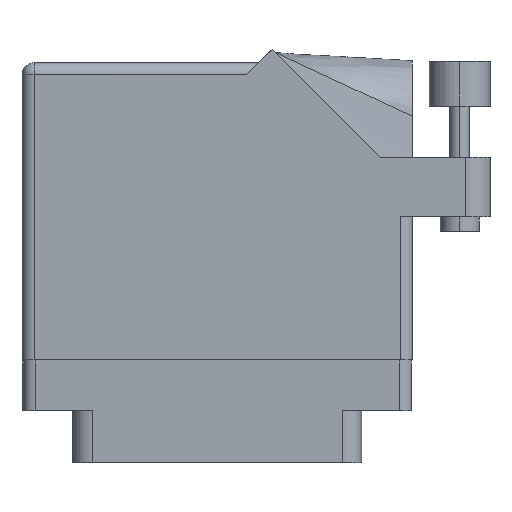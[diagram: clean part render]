
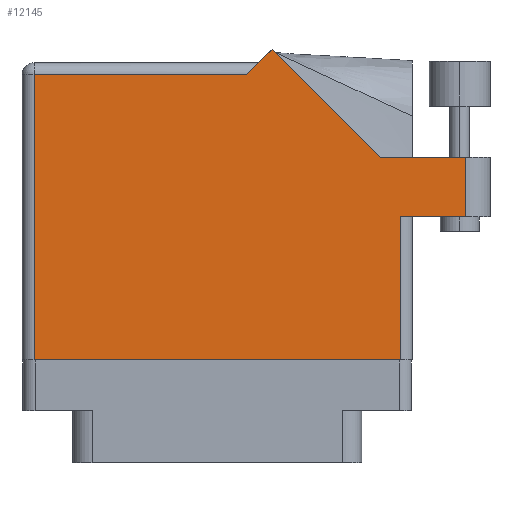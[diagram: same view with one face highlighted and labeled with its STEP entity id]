
A CAD part, front view. The second image highlights one B-rep face of the part: STEP entity #12145.
In plain terms, the highlighted face is planar.
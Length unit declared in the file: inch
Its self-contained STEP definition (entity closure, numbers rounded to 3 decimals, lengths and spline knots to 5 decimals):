
#22 = EDGE_CURVE ( 'NONE', #29785, #17915, #18561, .T. ) ;
#189 = VECTOR ( 'NONE', #18641, 39.37008 ) ;
#214 = EDGE_CURVE ( 'NONE', #4369, #27456, #34689, .T. ) ;
#499 = CARTESIAN_POINT ( 'NONE',  ( 1.155, 1.468, 0. ) ) ;
#653 = VECTOR ( 'NONE', #2954, 39.37008 ) ;
#1097 = EDGE_CURVE ( 'NONE', #23793, #20524, #4076, .T. ) ;
#1210 = DIRECTION ( 'NONE',  ( -0.707, 0.707, 0. ) ) ;
#1542 = LINE ( 'NONE', #4793, #31627 ) ;
#1667 = ORIENTED_EDGE ( 'NONE', *, *, #27074, .T. ) ;
#2067 = DIRECTION ( 'NONE',  ( -1., 0., 0. ) ) ;
#2954 = DIRECTION ( 'NONE',  ( 0., 1., 0. ) ) ;
#3857 = EDGE_CURVE ( 'NONE', #32932, #30769, #30040, .T. ) ;
#4076 = LINE ( 'NONE', #8030, #653 ) ;
#4369 = VERTEX_POINT ( 'NONE', #22173 ) ;
#4793 = CARTESIAN_POINT ( 'NONE',  ( 0., 1.468, 0. ) ) ;
#6001 = AXIS2_PLACEMENT_3D ( 'NONE', #27174, #24192, #10722 ) ;
#6480 = ORIENTED_EDGE ( 'NONE', *, *, #1097, .T. ) ;
#6632 = ORIENTED_EDGE ( 'NONE', *, *, #27361, .T. ) ;
#6941 = CARTESIAN_POINT ( 'NONE',  ( 0.062, 1.468, 0. ) ) ;
#8030 = CARTESIAN_POINT ( 'NONE',  ( 2.285, 1.044, 0. ) ) ;
#8979 = EDGE_CURVE ( 'NONE', #17915, #32932, #12781, .T. ) ;
#9488 = CARTESIAN_POINT ( 'NONE',  ( 1.28771, 1.60071, 0. ) ) ;
#10154 = ORIENTED_EDGE ( 'NONE', *, *, #3857, .T. ) ;
#10722 = DIRECTION ( 'NONE',  ( -1., 0., 0. ) ) ;
#11071 = DIRECTION ( 'NONE',  ( 0., -1., 0. ) ) ;
#11701 = ORIENTED_EDGE ( 'NONE', *, *, #8979, .T. ) ;
#12088 = DIRECTION ( 'NONE',  ( 1., 0., 0. ) ) ;
#12145 = ADVANCED_FACE ( 'NONE', ( #30816 ), #26584, .F. ) ;
#12781 = LINE ( 'NONE', #18675, #31869 ) ;
#14304 = CARTESIAN_POINT ( 'NONE',  ( 2.41, 1.044, 0. ) ) ;
#14750 = ORIENTED_EDGE ( 'NONE', *, *, #30734, .T. ) ;
#14753 = VERTEX_POINT ( 'NONE', #499 ) ;
#14985 = DIRECTION ( 'NONE',  ( 0., 1., 0. ) ) ;
#15980 = CARTESIAN_POINT ( 'NONE',  ( 0.062, 0., 0. ) ) ;
#16322 = VECTOR ( 'NONE', #12088, 39.37008 ) ;
#16423 = LINE ( 'NONE', #14304, #21892 ) ;
#17915 = VERTEX_POINT ( 'NONE', #15980 ) ;
#18112 = ORIENTED_EDGE ( 'NONE', *, *, #22, .T. ) ;
#18473 = ORIENTED_EDGE ( 'NONE', *, *, #29672, .T. ) ;
#18519 = CARTESIAN_POINT ( 'NONE',  ( 1.948, 0., 0. ) ) ;
#18561 = LINE ( 'NONE', #32545, #33428 ) ;
#18641 = DIRECTION ( 'NONE',  ( -0.707, -0.707, 0. ) ) ;
#18675 = CARTESIAN_POINT ( 'NONE',  ( 0., 0., 0. ) ) ;
#18954 = VECTOR ( 'NONE', #1210, 39.37008 ) ;
#18982 = CARTESIAN_POINT ( 'NONE',  ( 1.217, 1.53, 0. ) ) ;
#20366 = EDGE_LOOP ( 'NONE', ( #6632, #6480, #18473, #31180, #14750, #1667, #18112, #11701, #10154 ) ) ;
#20524 = VERTEX_POINT ( 'NONE', #21796 ) ;
#21736 = CARTESIAN_POINT ( 'NONE',  ( 2.285, 0.737, 0. ) ) ;
#21796 = CARTESIAN_POINT ( 'NONE',  ( 2.285, 1.044, 0. ) ) ;
#21892 = VECTOR ( 'NONE', #30542, 39.37008 ) ;
#22173 = CARTESIAN_POINT ( 'NONE',  ( 1.84442, 1.044, 0. ) ) ;
#23793 = VERTEX_POINT ( 'NONE', #21736 ) ;
#24074 = VECTOR ( 'NONE', #14985, 39.37008 ) ;
#24192 = DIRECTION ( 'NONE',  ( 0., 0., -1. ) ) ;
#25322 = CARTESIAN_POINT ( 'NONE',  ( 2.01, 0.737, 0. ) ) ;
#25728 = CARTESIAN_POINT ( 'NONE',  ( 1.84442, 1.044, 0. ) ) ;
#26508 = DIRECTION ( 'NONE',  ( 1., 0., 0. ) ) ;
#26584 = PLANE ( 'NONE',  #6001 ) ;
#27074 = EDGE_CURVE ( 'NONE', #14753, #29785, #1542, .T. ) ;
#27174 = CARTESIAN_POINT ( 'NONE',  ( 0., 1.53, 0. ) ) ;
#27361 = EDGE_CURVE ( 'NONE', #30769, #23793, #33756, .T. ) ;
#27456 = VERTEX_POINT ( 'NONE', #9488 ) ;
#29549 = CARTESIAN_POINT ( 'NONE',  ( 1.948, 0.737, 0. ) ) ;
#29672 = EDGE_CURVE ( 'NONE', #20524, #4369, #16423, .T. ) ;
#29785 = VERTEX_POINT ( 'NONE', #6941 ) ;
#30040 = LINE ( 'NONE', #33644, #24074 ) ;
#30309 = LINE ( 'NONE', #18982, #189 ) ;
#30542 = DIRECTION ( 'NONE',  ( -1., 0., 0. ) ) ;
#30734 = EDGE_CURVE ( 'NONE', #27456, #14753, #30309, .T. ) ;
#30769 = VERTEX_POINT ( 'NONE', #29549 ) ;
#30816 = FACE_OUTER_BOUND ( 'NONE', #20366, .T. ) ;
#31180 = ORIENTED_EDGE ( 'NONE', *, *, #214, .T. ) ;
#31627 = VECTOR ( 'NONE', #2067, 39.37008 ) ;
#31869 = VECTOR ( 'NONE', #26508, 39.37008 ) ;
#32545 = CARTESIAN_POINT ( 'NONE',  ( 0.062, 0., 0. ) ) ;
#32932 = VERTEX_POINT ( 'NONE', #18519 ) ;
#33428 = VECTOR ( 'NONE', #11071, 39.37008 ) ;
#33644 = CARTESIAN_POINT ( 'NONE',  ( 1.948, 0.737, 0. ) ) ;
#33756 = LINE ( 'NONE', #25322, #16322 ) ;
#34689 = LINE ( 'NONE', #25728, #18954 ) ;
